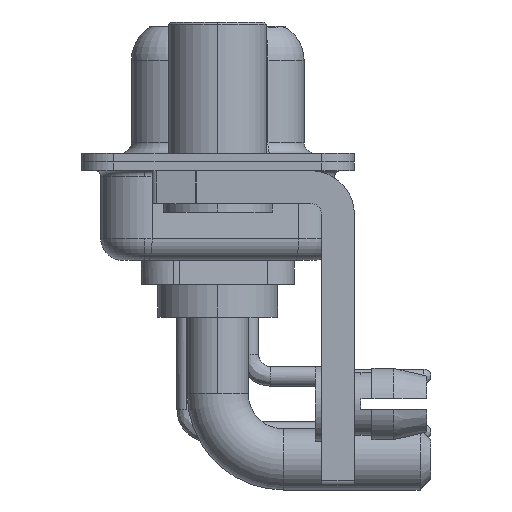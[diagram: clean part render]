
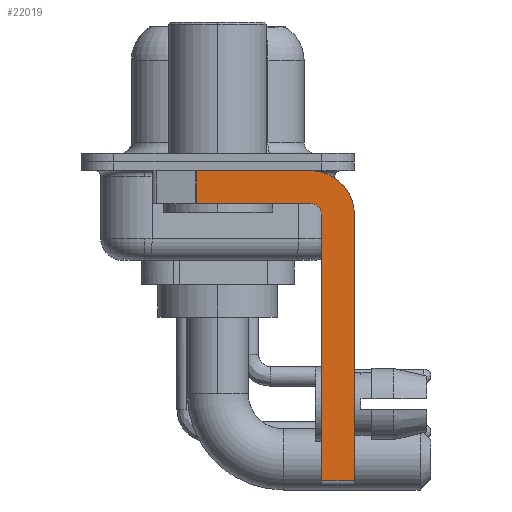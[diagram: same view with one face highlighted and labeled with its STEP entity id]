
A CAD part, left-side view. The second image highlights one B-rep face of the part: STEP entity #22019.
In plain terms, the highlighted planar face has unit normal (-1, 0, 0).
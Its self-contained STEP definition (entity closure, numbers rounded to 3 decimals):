
#1308 = DIRECTION ( 'NONE',  ( 0., 0., 1. ) ) ;
#1864 = VERTEX_POINT ( 'NONE', #9896 ) ;
#2410 = EDGE_CURVE ( 'NONE', #16540, #14373, #21463, .T. ) ;
#2540 = DIRECTION ( 'NONE',  ( 0., -1., 0. ) ) ;
#3172 = CARTESIAN_POINT ( 'NONE',  ( -2.9, -4.25, -2.4 ) ) ;
#4774 = DIRECTION ( 'NONE',  ( -1., 0., 0. ) ) ;
#5001 = CARTESIAN_POINT ( 'NONE',  ( -2.9, -4.75, -2.4 ) ) ;
#5465 = ORIENTED_EDGE ( 'NONE', *, *, #7121, .T. ) ;
#5680 = ORIENTED_EDGE ( 'NONE', *, *, #23481, .F. ) ;
#6328 = ORIENTED_EDGE ( 'NONE', *, *, #21109, .F. ) ;
#7038 = DIRECTION ( 'NONE',  ( 0., 0., -1. ) ) ;
#7121 = EDGE_CURVE ( 'NONE', #1864, #14373, #20222, .T. ) ;
#7776 = EDGE_CURVE ( 'NONE', #7948, #22983, #9480, .T. ) ;
#7948 = VERTEX_POINT ( 'NONE', #21066 ) ;
#8320 = DIRECTION ( 'NONE',  ( 0., 0., -1. ) ) ;
#8521 = DIRECTION ( 'NONE',  ( 0., 1., 0. ) ) ;
#9110 = DIRECTION ( 'NONE',  ( 0., 0., 1. ) ) ;
#9142 = FACE_OUTER_BOUND ( 'NONE', #12945, .T. ) ;
#9269 = PLANE ( 'NONE',  #14457 ) ;
#9480 = LINE ( 'NONE', #10953, #23921 ) ;
#9726 = ORIENTED_EDGE ( 'NONE', *, *, #21074, .F. ) ;
#9870 = DIRECTION ( 'NONE',  ( 0., -1., 0. ) ) ;
#9896 = CARTESIAN_POINT ( 'NONE',  ( -2.9, 0.978, -0.4 ) ) ;
#10476 = CARTESIAN_POINT ( 'NONE',  ( -2.9, -4.25, -1.9 ) ) ;
#10822 = CARTESIAN_POINT ( 'NONE',  ( -2.9, -6.25, -14.55 ) ) ;
#10953 = CARTESIAN_POINT ( 'NONE',  ( -2.9, -4.75, -14.8 ) ) ;
#11102 = DIRECTION ( 'NONE',  ( 1., 0., 0. ) ) ;
#11314 = VECTOR ( 'NONE', #2540, 1000. ) ;
#11847 = CARTESIAN_POINT ( 'NONE',  ( -2.9, -4.25, -14.55 ) ) ;
#11886 = LINE ( 'NONE', #19399, #11314 ) ;
#12808 = DIRECTION ( 'NONE',  ( 0., 0., -1. ) ) ;
#12945 = EDGE_LOOP ( 'NONE', ( #6328, #5465, #13610, #17289, #20031, #16251, #9726, #5680 ) ) ;
#13330 = CARTESIAN_POINT ( 'NONE',  ( -2.9, -4.25, -1.9 ) ) ;
#13384 = VERTEX_POINT ( 'NONE', #13434 ) ;
#13434 = CARTESIAN_POINT ( 'NONE',  ( -2.9, -4.25, -0.4 ) ) ;
#13610 = ORIENTED_EDGE ( 'NONE', *, *, #2410, .F. ) ;
#14147 = VERTEX_POINT ( 'NONE', #18336 ) ;
#14159 = CARTESIAN_POINT ( 'NONE',  ( -2.9, 0.978, -1.9 ) ) ;
#14285 = CIRCLE ( 'NONE', #20610, 0.5 ) ;
#14373 = VERTEX_POINT ( 'NONE', #24267 ) ;
#14457 = AXIS2_PLACEMENT_3D ( 'NONE', #14903, #11102, #12808 ) ;
#14903 = CARTESIAN_POINT ( 'NONE',  ( -2.9, -4.25, -2.4 ) ) ;
#16251 = ORIENTED_EDGE ( 'NONE', *, *, #24066, .T. ) ;
#16540 = VERTEX_POINT ( 'NONE', #13330 ) ;
#16866 = CARTESIAN_POINT ( 'NONE',  ( -2.9, -4.25, -2.4 ) ) ;
#17289 = ORIENTED_EDGE ( 'NONE', *, *, #17528, .F. ) ;
#17528 = EDGE_CURVE ( 'NONE', #22983, #16540, #14285, .T. ) ;
#17780 = CARTESIAN_POINT ( 'NONE',  ( -2.9, -6.25, -2.4 ) ) ;
#18336 = CARTESIAN_POINT ( 'NONE',  ( -2.9, -6.25, -2.4 ) ) ;
#18723 = DIRECTION ( 'NONE',  ( 1., 0., 0. ) ) ;
#19280 = LINE ( 'NONE', #17780, #21153 ) ;
#19399 = CARTESIAN_POINT ( 'NONE',  ( -2.9, 3., -0.4 ) ) ;
#19582 = AXIS2_PLACEMENT_3D ( 'NONE', #16866, #18723, #20454 ) ;
#20031 = ORIENTED_EDGE ( 'NONE', *, *, #7776, .F. ) ;
#20222 = LINE ( 'NONE', #14159, #20744 ) ;
#20379 = CIRCLE ( 'NONE', #19582, 2. ) ;
#20454 = DIRECTION ( 'NONE',  ( 0., 0., -1. ) ) ;
#20610 = AXIS2_PLACEMENT_3D ( 'NONE', #3172, #4774, #1308 ) ;
#20744 = VECTOR ( 'NONE', #7038, 1000. ) ;
#21066 = CARTESIAN_POINT ( 'NONE',  ( -2.9, -4.75, -14.55 ) ) ;
#21074 = EDGE_CURVE ( 'NONE', #14147, #21520, #19280, .T. ) ;
#21109 = EDGE_CURVE ( 'NONE', #1864, #13384, #11886, .T. ) ;
#21153 = VECTOR ( 'NONE', #8320, 1000. ) ;
#21463 = LINE ( 'NONE', #10476, #22992 ) ;
#21520 = VERTEX_POINT ( 'NONE', #10822 ) ;
#22019 = ADVANCED_FACE ( 'NONE', ( #9142 ), #9269, .F. ) ;
#22983 = VERTEX_POINT ( 'NONE', #5001 ) ;
#22992 = VECTOR ( 'NONE', #8521, 1000. ) ;
#23202 = LINE ( 'NONE', #11847, #23566 ) ;
#23481 = EDGE_CURVE ( 'NONE', #13384, #14147, #20379, .T. ) ;
#23566 = VECTOR ( 'NONE', #9870, 1000. ) ;
#23921 = VECTOR ( 'NONE', #9110, 1000. ) ;
#24066 = EDGE_CURVE ( 'NONE', #7948, #21520, #23202, .T. ) ;
#24267 = CARTESIAN_POINT ( 'NONE',  ( -2.9, 0.978, -1.9 ) ) ;
